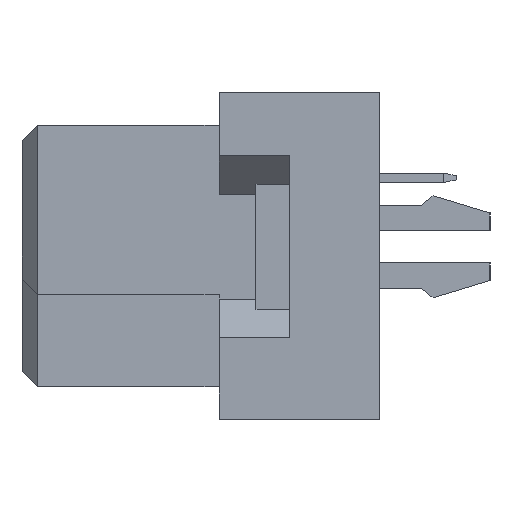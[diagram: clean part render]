
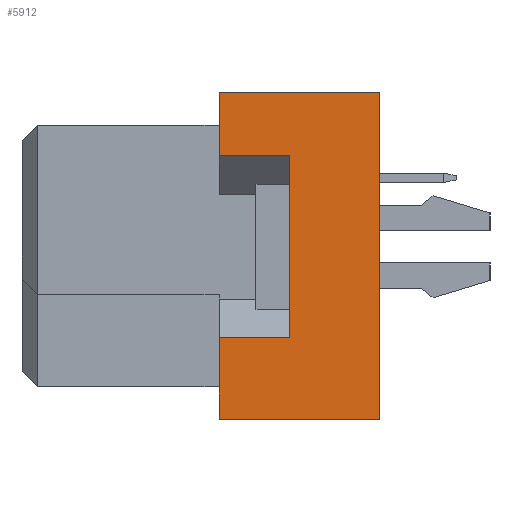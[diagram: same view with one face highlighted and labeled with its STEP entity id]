
A CAD part, left-side view. The second image highlights one B-rep face of the part: STEP entity #5912.
In plain terms, the highlighted planar face has unit normal (-1, 0, 0).
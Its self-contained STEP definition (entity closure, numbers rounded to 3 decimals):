
#2 = EDGE_CURVE ( 'NONE', #2364, #25751, #27011, .T. ) ;
#704 = LINE ( 'NONE', #27084, #31229 ) ;
#1151 = CARTESIAN_POINT ( 'NONE',  ( -47.5, -11.6, -5.3 ) ) ;
#1667 = CARTESIAN_POINT ( 'NONE',  ( -47.5, -6.4, -5.3 ) ) ;
#2047 = CARTESIAN_POINT ( 'NONE',  ( -47.5, -6.4, 3.25 ) ) ;
#2364 = VERTEX_POINT ( 'NONE', #19408 ) ;
#2420 = CARTESIAN_POINT ( 'NONE',  ( -47.5, -11.6, 5.3 ) ) ;
#2918 = CARTESIAN_POINT ( 'NONE',  ( -47.5, -11.6, 5.3 ) ) ;
#3081 = DIRECTION ( 'NONE',  ( 0., 0., 1. ) ) ;
#3913 = EDGE_CURVE ( 'NONE', #2364, #18750, #36961, .T. ) ;
#4909 = LINE ( 'NONE', #10795, #30279 ) ;
#4930 = ORIENTED_EDGE ( 'NONE', *, *, #17047, .F. ) ;
#5235 = ORIENTED_EDGE ( 'NONE', *, *, #36000, .F. ) ;
#5410 = FACE_OUTER_BOUND ( 'NONE', #25692, .T. ) ;
#5912 = ADVANCED_FACE ( 'NONE', ( #5410 ), #17404, .T. ) ;
#5924 = ORIENTED_EDGE ( 'NONE', *, *, #6598, .F. ) ;
#6139 = DIRECTION ( 'NONE',  ( 0., 0., 1. ) ) ;
#6598 = EDGE_CURVE ( 'NONE', #20303, #35022, #37975, .T. ) ;
#9558 = CARTESIAN_POINT ( 'NONE',  ( -47.5, -6.4, 5.3 ) ) ;
#9717 = DIRECTION ( 'NONE',  ( 0., 0., 1. ) ) ;
#10491 = CARTESIAN_POINT ( 'NONE',  ( -47.5, -8.7, 3.25 ) ) ;
#10565 = DIRECTION ( 'NONE',  ( 0., 1., 0. ) ) ;
#10795 = CARTESIAN_POINT ( 'NONE',  ( -47.5, -8.7, -2.65 ) ) ;
#12266 = ORIENTED_EDGE ( 'NONE', *, *, #20805, .T. ) ;
#12726 = VECTOR ( 'NONE', #10565, 1000. ) ;
#12811 = EDGE_CURVE ( 'NONE', #20303, #30691, #4909, .T. ) ;
#15425 = AXIS2_PLACEMENT_3D ( 'NONE', #26463, #38454, #9717 ) ;
#15708 = DIRECTION ( 'NONE',  ( 0., 1., 0. ) ) ;
#16452 = CARTESIAN_POINT ( 'NONE',  ( -47.5, -11.6, 5.3 ) ) ;
#17047 = EDGE_CURVE ( 'NONE', #33354, #17053, #704, .T. ) ;
#17053 = VERTEX_POINT ( 'NONE', #9558 ) ;
#17155 = VECTOR ( 'NONE', #34906, 1000. ) ;
#17404 = PLANE ( 'NONE',  #15425 ) ;
#17412 = CARTESIAN_POINT ( 'NONE',  ( -47.5, -8.7, 3.25 ) ) ;
#17789 = LINE ( 'NONE', #17412, #24975 ) ;
#18456 = EDGE_CURVE ( 'NONE', #18750, #30691, #22901, .T. ) ;
#18750 = VERTEX_POINT ( 'NONE', #36275 ) ;
#19408 = CARTESIAN_POINT ( 'NONE',  ( -47.5, -11.6, -5.3 ) ) ;
#20303 = VERTEX_POINT ( 'NONE', #30309 ) ;
#20805 = EDGE_CURVE ( 'NONE', #25751, #17053, #28865, .T. ) ;
#22901 = LINE ( 'NONE', #1667, #17155 ) ;
#23026 = CARTESIAN_POINT ( 'NONE',  ( -47.5, -8.7, -2.65 ) ) ;
#24975 = VECTOR ( 'NONE', #29802, 1000. ) ;
#25692 = EDGE_LOOP ( 'NONE', ( #30222, #31678, #30725, #32752, #12266, #4930, #5235, #5924 ) ) ;
#25700 = VECTOR ( 'NONE', #6139, 1000. ) ;
#25751 = VERTEX_POINT ( 'NONE', #2918 ) ;
#26463 = CARTESIAN_POINT ( 'NONE',  ( -47.5, -11.6, 5.3 ) ) ;
#27011 = LINE ( 'NONE', #2420, #25700 ) ;
#27084 = CARTESIAN_POINT ( 'NONE',  ( -47.5, -6.4, -5.3 ) ) ;
#28500 = VECTOR ( 'NONE', #15708, 1000. ) ;
#28865 = LINE ( 'NONE', #16452, #12726 ) ;
#29802 = DIRECTION ( 'NONE',  ( 0., 1., 0. ) ) ;
#30222 = ORIENTED_EDGE ( 'NONE', *, *, #12811, .T. ) ;
#30279 = VECTOR ( 'NONE', #31281, 1000. ) ;
#30309 = CARTESIAN_POINT ( 'NONE',  ( -47.5, -8.7, -2.65 ) ) ;
#30691 = VERTEX_POINT ( 'NONE', #31276 ) ;
#30725 = ORIENTED_EDGE ( 'NONE', *, *, #3913, .F. ) ;
#31229 = VECTOR ( 'NONE', #3081, 1000. ) ;
#31276 = CARTESIAN_POINT ( 'NONE',  ( -47.5, -6.4, -2.65 ) ) ;
#31281 = DIRECTION ( 'NONE',  ( 0., 1., 0. ) ) ;
#31316 = DIRECTION ( 'NONE',  ( 0., 0., 1. ) ) ;
#31678 = ORIENTED_EDGE ( 'NONE', *, *, #18456, .F. ) ;
#32466 = VECTOR ( 'NONE', #31316, 1000. ) ;
#32752 = ORIENTED_EDGE ( 'NONE', *, *, #2, .T. ) ;
#33354 = VERTEX_POINT ( 'NONE', #2047 ) ;
#34906 = DIRECTION ( 'NONE',  ( 0., 0., 1. ) ) ;
#35022 = VERTEX_POINT ( 'NONE', #10491 ) ;
#36000 = EDGE_CURVE ( 'NONE', #35022, #33354, #17789, .T. ) ;
#36275 = CARTESIAN_POINT ( 'NONE',  ( -47.5, -6.4, -5.3 ) ) ;
#36961 = LINE ( 'NONE', #1151, #28500 ) ;
#37975 = LINE ( 'NONE', #23026, #32466 ) ;
#38454 = DIRECTION ( 'NONE',  ( -1., 0., 0. ) ) ;
